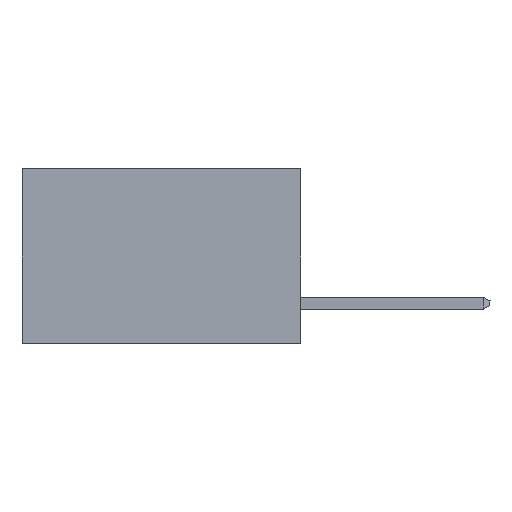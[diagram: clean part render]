
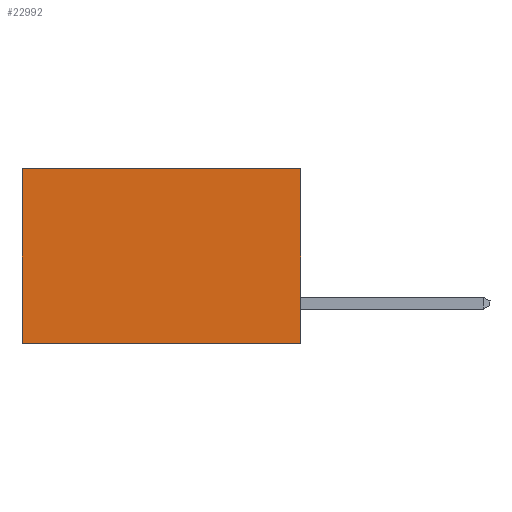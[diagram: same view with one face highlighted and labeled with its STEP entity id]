
A CAD part, left-side view. The second image highlights one B-rep face of the part: STEP entity #22992.
In plain terms, the highlighted planar face has unit normal (-1, 0, 0).
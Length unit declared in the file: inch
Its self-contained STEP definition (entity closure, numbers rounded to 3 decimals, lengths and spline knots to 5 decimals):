
#659 = EDGE_LOOP ( 'NONE', ( #10681, #2483, #3064, #26933 ) ) ;
#833 = DIRECTION ( 'NONE',  ( 0., 1., 0. ) ) ;
#1315 = AXIS2_PLACEMENT_3D ( 'NONE', #22283, #18344, #5640 ) ;
#2117 = VECTOR ( 'NONE', #10759, 39.37008 ) ;
#2135 = VERTEX_POINT ( 'NONE', #14489 ) ;
#2249 = CARTESIAN_POINT ( 'NONE',  ( 0.277, 0., 0. ) ) ;
#2483 = ORIENTED_EDGE ( 'NONE', *, *, #23236, .F. ) ;
#2684 = CARTESIAN_POINT ( 'NONE',  ( 0.277, 0.59, 0. ) ) ;
#3064 = ORIENTED_EDGE ( 'NONE', *, *, #15625, .F. ) ;
#4204 = VECTOR ( 'NONE', #833, 39.37008 ) ;
#4307 = VECTOR ( 'NONE', #7126, 39.37008 ) ;
#4446 = VERTEX_POINT ( 'NONE', #14802 ) ;
#4785 = CARTESIAN_POINT ( 'NONE',  ( 0.277, 0.59, -0.37 ) ) ;
#4837 = EDGE_CURVE ( 'NONE', #2135, #10897, #10840, .T. ) ;
#5640 = DIRECTION ( 'NONE',  ( 0., 0., -1. ) ) ;
#5902 = EDGE_CURVE ( 'NONE', #10897, #4446, #15752, .T. ) ;
#6443 = LINE ( 'NONE', #13548, #16996 ) ;
#7126 = DIRECTION ( 'NONE',  ( 0., 0., -1. ) ) ;
#9824 = DIRECTION ( 'NONE',  ( 0., 0., -1. ) ) ;
#10021 = PLANE ( 'NONE',  #1315 ) ;
#10681 = ORIENTED_EDGE ( 'NONE', *, *, #5902, .T. ) ;
#10759 = DIRECTION ( 'NONE',  ( 0., 1., 0. ) ) ;
#10840 = LINE ( 'NONE', #2249, #4204 ) ;
#10897 = VERTEX_POINT ( 'NONE', #2684 ) ;
#12821 = FACE_OUTER_BOUND ( 'NONE', #659, .T. ) ;
#13548 = CARTESIAN_POINT ( 'NONE',  ( 0.277, 0., -0.37 ) ) ;
#13737 = LINE ( 'NONE', #17317, #2117 ) ;
#14489 = CARTESIAN_POINT ( 'NONE',  ( 0.277, 0., 0. ) ) ;
#14802 = CARTESIAN_POINT ( 'NONE',  ( 0.277, 0.59, -0.37 ) ) ;
#15625 = EDGE_CURVE ( 'NONE', #2135, #20509, #6443, .T. ) ;
#15752 = LINE ( 'NONE', #4785, #4307 ) ;
#16996 = VECTOR ( 'NONE', #9824, 39.37008 ) ;
#17317 = CARTESIAN_POINT ( 'NONE',  ( 0.277, 0., -0.37 ) ) ;
#18344 = DIRECTION ( 'NONE',  ( 1., 0., 0. ) ) ;
#20509 = VERTEX_POINT ( 'NONE', #26383 ) ;
#22283 = CARTESIAN_POINT ( 'NONE',  ( 0.277, 0., -0.37 ) ) ;
#22992 = ADVANCED_FACE ( 'NONE', ( #12821 ), #10021, .F. ) ;
#23236 = EDGE_CURVE ( 'NONE', #20509, #4446, #13737, .T. ) ;
#26383 = CARTESIAN_POINT ( 'NONE',  ( 0.277, 0., -0.37 ) ) ;
#26933 = ORIENTED_EDGE ( 'NONE', *, *, #4837, .T. ) ;
